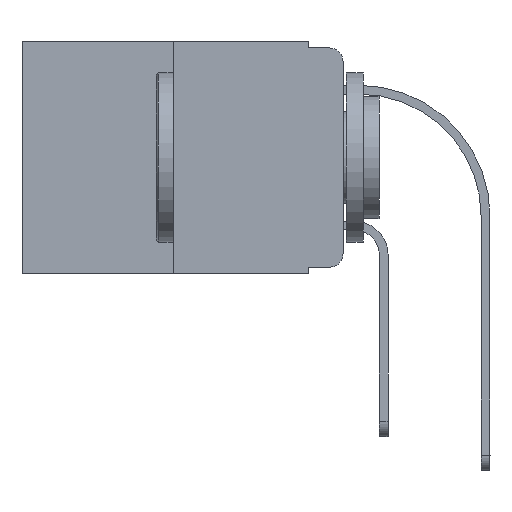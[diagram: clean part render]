
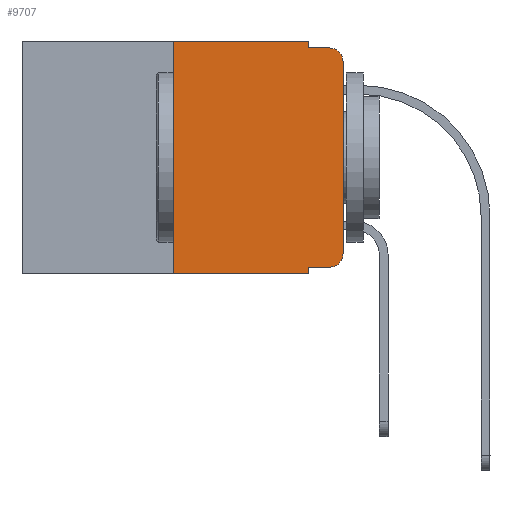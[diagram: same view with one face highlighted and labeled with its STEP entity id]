
A CAD part, left-side view. The second image highlights one B-rep face of the part: STEP entity #9707.
In plain terms, the highlighted planar face has unit normal (-1, 0, 0).
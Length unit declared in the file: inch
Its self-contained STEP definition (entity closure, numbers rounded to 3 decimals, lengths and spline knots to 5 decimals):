
#21 = EDGE_CURVE ( 'NONE', #1051, #6158, #5887, .T. ) ;
#51 = AXIS2_PLACEMENT_3D ( 'NONE', #9535, #3592, #14572 ) ;
#130 = AXIS2_PLACEMENT_3D ( 'NONE', #3818, #8606, #11989 ) ;
#150 = CARTESIAN_POINT ( 'NONE',  ( 0., 0.473, -0.343 ) ) ;
#177 = PLANE ( 'NONE',  #130 ) ;
#403 = FACE_OUTER_BOUND ( 'NONE', #6323, .T. ) ;
#471 = CARTESIAN_POINT ( 'NONE',  ( 0., 0.051, 0. ) ) ;
#495 = ORIENTED_EDGE ( 'NONE', *, *, #5875, .T. ) ;
#898 = CARTESIAN_POINT ( 'NONE',  ( 0., 0.02, -0.01 ) ) ;
#962 = ORIENTED_EDGE ( 'NONE', *, *, #6644, .T. ) ;
#1051 = VERTEX_POINT ( 'NONE', #12707 ) ;
#1062 = CARTESIAN_POINT ( 'NONE',  ( 0., 0.051, -0.333 ) ) ;
#1128 = VERTEX_POINT ( 'NONE', #898 ) ;
#1609 = VECTOR ( 'NONE', #4818, 39.37008 ) ;
#1730 = CARTESIAN_POINT ( 'NONE',  ( 0., 0.25, -0.343 ) ) ;
#2034 = CIRCLE ( 'NONE', #51, 0.02 ) ;
#2083 = VECTOR ( 'NONE', #15375, 39.37008 ) ;
#3242 = DIRECTION ( 'NONE',  ( 0., 0., -1. ) ) ;
#3308 = VERTEX_POINT ( 'NONE', #14396 ) ;
#3592 = DIRECTION ( 'NONE',  ( -1., 0., 0. ) ) ;
#3680 = VECTOR ( 'NONE', #12592, 39.37008 ) ;
#3818 = CARTESIAN_POINT ( 'NONE',  ( 0., 0.473, 0. ) ) ;
#4447 = EDGE_CURVE ( 'NONE', #9755, #13740, #9495, .T. ) ;
#4746 = LINE ( 'NONE', #8356, #1609 ) ;
#4818 = DIRECTION ( 'NONE',  ( 0., 0., 1. ) ) ;
#4885 = EDGE_CURVE ( 'NONE', #3308, #6241, #5320, .T. ) ;
#4988 = LINE ( 'NONE', #13610, #3680 ) ;
#5002 = EDGE_CURVE ( 'NONE', #13039, #9877, #5550, .T. ) ;
#5173 = CARTESIAN_POINT ( 'NONE',  ( 0., 0.473, 0. ) ) ;
#5289 = CARTESIAN_POINT ( 'NONE',  ( 0., 0.051, -0.343 ) ) ;
#5320 = LINE ( 'NONE', #5173, #6112 ) ;
#5348 = EDGE_CURVE ( 'NONE', #13039, #13740, #4988, .T. ) ;
#5550 = LINE ( 'NONE', #9008, #15359 ) ;
#5875 = EDGE_CURVE ( 'NONE', #9877, #1051, #7026, .T. ) ;
#5887 = LINE ( 'NONE', #9474, #8665 ) ;
#6112 = VECTOR ( 'NONE', #6436, 39.37008 ) ;
#6158 = VERTEX_POINT ( 'NONE', #8321 ) ;
#6241 = VERTEX_POINT ( 'NONE', #9943 ) ;
#6318 = DIRECTION ( 'NONE',  ( 0., 0., -1. ) ) ;
#6323 = EDGE_LOOP ( 'NONE', ( #8206, #962, #13909, #15172, #14580, #12856, #7451, #10866, #7160, #495 ) ) ;
#6436 = DIRECTION ( 'NONE',  ( 0., -1., 0. ) ) ;
#6644 = EDGE_CURVE ( 'NONE', #6158, #1128, #2034, .T. ) ;
#6778 = LINE ( 'NONE', #11281, #7040 ) ;
#7026 = CIRCLE ( 'NONE', #8785, 0.02 ) ;
#7040 = VECTOR ( 'NONE', #7882, 39.37008 ) ;
#7160 = ORIENTED_EDGE ( 'NONE', *, *, #5002, .T. ) ;
#7334 = EDGE_CURVE ( 'NONE', #14156, #1128, #6778, .T. ) ;
#7451 = ORIENTED_EDGE ( 'NONE', *, *, #4447, .T. ) ;
#7882 = DIRECTION ( 'NONE',  ( 0., -1., 0. ) ) ;
#8206 = ORIENTED_EDGE ( 'NONE', *, *, #21, .T. ) ;
#8321 = CARTESIAN_POINT ( 'NONE',  ( 0., 0., -0.03 ) ) ;
#8356 = CARTESIAN_POINT ( 'NONE',  ( 0., 0.25, 0. ) ) ;
#8406 = EDGE_CURVE ( 'NONE', #6241, #14156, #14553, .T. ) ;
#8606 = DIRECTION ( 'NONE',  ( 1., 0., 0. ) ) ;
#8664 = CARTESIAN_POINT ( 'NONE',  ( 0., 0.051, -0.01 ) ) ;
#8665 = VECTOR ( 'NONE', #9550, 39.37008 ) ;
#8785 = AXIS2_PLACEMENT_3D ( 'NONE', #10121, #14056, #3242 ) ;
#8819 = VECTOR ( 'NONE', #6318, 39.37008 ) ;
#9008 = CARTESIAN_POINT ( 'NONE',  ( 0., 0.051, -0.333 ) ) ;
#9474 = CARTESIAN_POINT ( 'NONE',  ( 0., 0., 0. ) ) ;
#9495 = LINE ( 'NONE', #150, #2083 ) ;
#9535 = CARTESIAN_POINT ( 'NONE',  ( 0., 0.02, -0.03 ) ) ;
#9550 = DIRECTION ( 'NONE',  ( 0., 0., 1. ) ) ;
#9707 = ADVANCED_FACE ( 'NONE', ( #403 ), #177, .F. ) ;
#9755 = VERTEX_POINT ( 'NONE', #1730 ) ;
#9877 = VERTEX_POINT ( 'NONE', #14878 ) ;
#9943 = CARTESIAN_POINT ( 'NONE',  ( 0., 0.051, 0. ) ) ;
#10121 = CARTESIAN_POINT ( 'NONE',  ( 0., 0.02, -0.313 ) ) ;
#10866 = ORIENTED_EDGE ( 'NONE', *, *, #5348, .F. ) ;
#11281 = CARTESIAN_POINT ( 'NONE',  ( 0., 0.051, -0.01 ) ) ;
#11989 = DIRECTION ( 'NONE',  ( 0., 0., -1. ) ) ;
#12592 = DIRECTION ( 'NONE',  ( 0., 0., -1. ) ) ;
#12707 = CARTESIAN_POINT ( 'NONE',  ( 0., 0., -0.313 ) ) ;
#12742 = EDGE_CURVE ( 'NONE', #9755, #3308, #4746, .T. ) ;
#12856 = ORIENTED_EDGE ( 'NONE', *, *, #12742, .F. ) ;
#13039 = VERTEX_POINT ( 'NONE', #1062 ) ;
#13610 = CARTESIAN_POINT ( 'NONE',  ( 0., 0.051, 0. ) ) ;
#13740 = VERTEX_POINT ( 'NONE', #5289 ) ;
#13909 = ORIENTED_EDGE ( 'NONE', *, *, #7334, .F. ) ;
#14056 = DIRECTION ( 'NONE',  ( -1., 0., 0. ) ) ;
#14156 = VERTEX_POINT ( 'NONE', #8664 ) ;
#14396 = CARTESIAN_POINT ( 'NONE',  ( 0., 0.25, 0. ) ) ;
#14553 = LINE ( 'NONE', #471, #8819 ) ;
#14572 = DIRECTION ( 'NONE',  ( 0., 0., -1. ) ) ;
#14580 = ORIENTED_EDGE ( 'NONE', *, *, #4885, .F. ) ;
#14878 = CARTESIAN_POINT ( 'NONE',  ( 0., 0.02, -0.333 ) ) ;
#15048 = DIRECTION ( 'NONE',  ( 0., -1., 0. ) ) ;
#15172 = ORIENTED_EDGE ( 'NONE', *, *, #8406, .F. ) ;
#15359 = VECTOR ( 'NONE', #15048, 39.37008 ) ;
#15375 = DIRECTION ( 'NONE',  ( 0., -1., 0. ) ) ;
